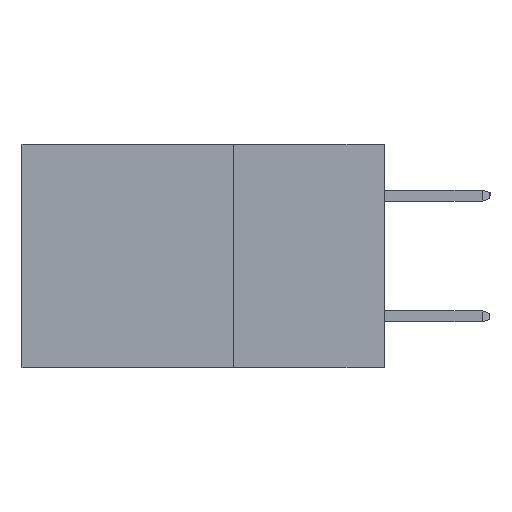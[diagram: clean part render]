
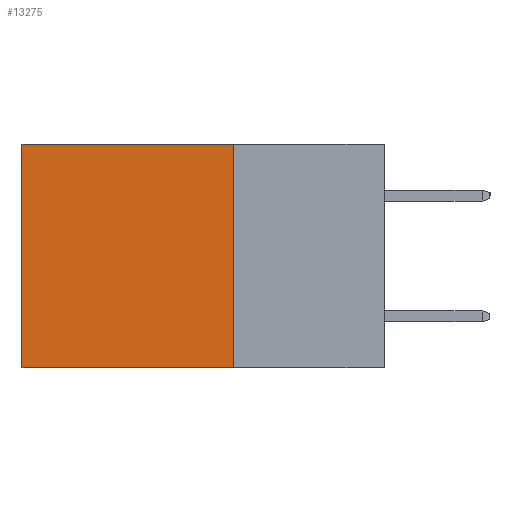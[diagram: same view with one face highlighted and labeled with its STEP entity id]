
A CAD part, left-side view. The second image highlights one B-rep face of the part: STEP entity #13275.
In plain terms, the highlighted planar face has unit normal (-1, 0, 0).
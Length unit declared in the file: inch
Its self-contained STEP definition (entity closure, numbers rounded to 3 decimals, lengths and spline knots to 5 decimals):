
#949 = DIRECTION ( 'NONE',  ( 0., 1., 0. ) ) ;
#1436 = VERTEX_POINT ( 'NONE', #10396 ) ;
#2298 = CARTESIAN_POINT ( 'NONE',  ( 0.2615, 0.25, -0.37 ) ) ;
#2689 = DIRECTION ( 'NONE',  ( 1., 0., 0. ) ) ;
#3196 = ORIENTED_EDGE ( 'NONE', *, *, #11215, .F. ) ;
#3609 = CARTESIAN_POINT ( 'NONE',  ( 0.2615, 0.25, -0.37 ) ) ;
#3964 = VERTEX_POINT ( 'NONE', #2298 ) ;
#4645 = CARTESIAN_POINT ( 'NONE',  ( 0.2615, 0.6, -0.37 ) ) ;
#5064 = CARTESIAN_POINT ( 'NONE',  ( 0.2615, 0.25, 0. ) ) ;
#5281 = CARTESIAN_POINT ( 'NONE',  ( 0.2615, 0.25, -0.37 ) ) ;
#5323 = VECTOR ( 'NONE', #17128, 39.37008 ) ;
#6256 = LINE ( 'NONE', #13060, #5323 ) ;
#6486 = ORIENTED_EDGE ( 'NONE', *, *, #16780, .F. ) ;
#7398 = CARTESIAN_POINT ( 'NONE',  ( 0.2615, 0.25, 0. ) ) ;
#7597 = LINE ( 'NONE', #3609, #17126 ) ;
#8095 = DIRECTION ( 'NONE',  ( 0., 0., -1. ) ) ;
#8591 = VECTOR ( 'NONE', #16764, 39.37008 ) ;
#9729 = VERTEX_POINT ( 'NONE', #7398 ) ;
#9862 = ORIENTED_EDGE ( 'NONE', *, *, #14744, .T. ) ;
#9882 = ORIENTED_EDGE ( 'NONE', *, *, #16462, .T. ) ;
#10396 = CARTESIAN_POINT ( 'NONE',  ( 0.2615, 0.6, 0. ) ) ;
#11173 = VECTOR ( 'NONE', #949, 39.37008 ) ;
#11215 = EDGE_CURVE ( 'NONE', #3964, #13610, #6256, .T. ) ;
#11364 = LINE ( 'NONE', #4645, #8591 ) ;
#12164 = FACE_OUTER_BOUND ( 'NONE', #13769, .T. ) ;
#13060 = CARTESIAN_POINT ( 'NONE',  ( 0.2615, 0.25, -0.37 ) ) ;
#13275 = ADVANCED_FACE ( 'NONE', ( #12164 ), #14745, .F. ) ;
#13610 = VERTEX_POINT ( 'NONE', #14970 ) ;
#13769 = EDGE_LOOP ( 'NONE', ( #9862, #3196, #6486, #9882 ) ) ;
#14744 = EDGE_CURVE ( 'NONE', #1436, #13610, #11364, .T. ) ;
#14745 = PLANE ( 'NONE',  #17035 ) ;
#14970 = CARTESIAN_POINT ( 'NONE',  ( 0.2615, 0.6, -0.37 ) ) ;
#15907 = DIRECTION ( 'NONE',  ( 0., 0., -1. ) ) ;
#16462 = EDGE_CURVE ( 'NONE', #9729, #1436, #17257, .T. ) ;
#16764 = DIRECTION ( 'NONE',  ( 0., 0., -1. ) ) ;
#16780 = EDGE_CURVE ( 'NONE', #9729, #3964, #7597, .T. ) ;
#17035 = AXIS2_PLACEMENT_3D ( 'NONE', #5281, #2689, #8095 ) ;
#17126 = VECTOR ( 'NONE', #15907, 39.37008 ) ;
#17128 = DIRECTION ( 'NONE',  ( 0., 1., 0. ) ) ;
#17257 = LINE ( 'NONE', #5064, #11173 ) ;
